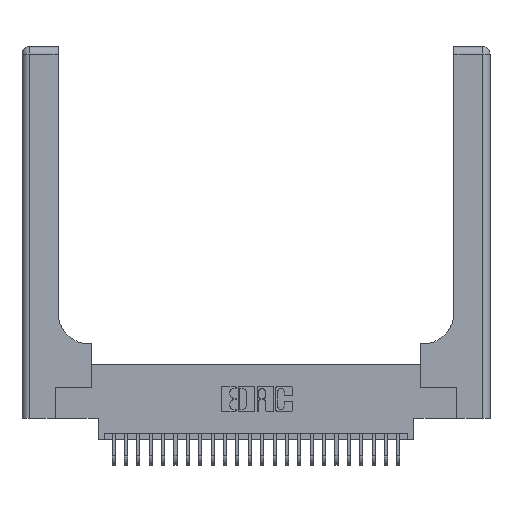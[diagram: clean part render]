
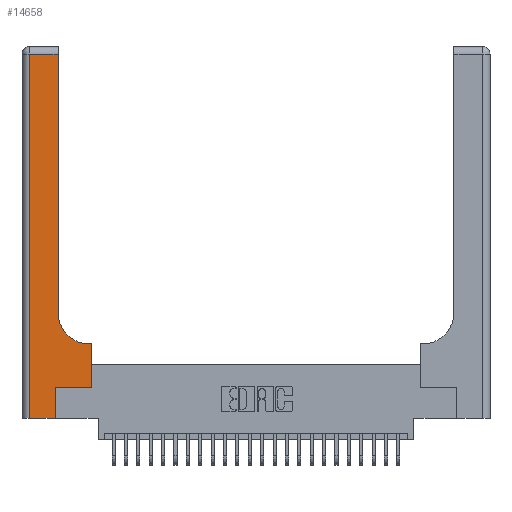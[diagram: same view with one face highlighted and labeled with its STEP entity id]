
A CAD part, top view. The second image highlights one B-rep face of the part: STEP entity #14658.
In plain terms, the highlighted planar face has unit normal (0, 0, 1).
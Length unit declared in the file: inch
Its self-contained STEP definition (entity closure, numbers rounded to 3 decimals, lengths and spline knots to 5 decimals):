
#450 = CARTESIAN_POINT ( 'NONE',  ( 0.06, 2.94, 0.37 ) ) ;
#3582 = LINE ( 'NONE', #26208, #14613 ) ;
#3914 = CARTESIAN_POINT ( 'NONE',  ( 0.2915, 2.94, 0.37 ) ) ;
#4185 = EDGE_CURVE ( 'NONE', #17432, #24767, #25683, .T. ) ;
#4216 = EDGE_CURVE ( 'NONE', #8321, #15777, #7664, .T. ) ;
#4225 = EDGE_CURVE ( 'NONE', #10453, #8321, #23656, .T. ) ;
#5013 = VERTEX_POINT ( 'NONE', #22377 ) ;
#6231 = ORIENTED_EDGE ( 'NONE', *, *, #25299, .T. ) ;
#6676 = DIRECTION ( 'NONE',  ( 0., 1., 0. ) ) ;
#6777 = CARTESIAN_POINT ( 'NONE',  ( 0.5415, 0.85, 0.37 ) ) ;
#6977 = VECTOR ( 'NONE', #6676, 39.37008 ) ;
#7330 = PLANE ( 'NONE',  #13040 ) ;
#7664 = LINE ( 'NONE', #8851, #6977 ) ;
#7935 = ORIENTED_EDGE ( 'NONE', *, *, #18161, .T. ) ;
#8321 = VERTEX_POINT ( 'NONE', #10564 ) ;
#8617 = VERTEX_POINT ( 'NONE', #15962 ) ;
#8851 = CARTESIAN_POINT ( 'NONE',  ( 0.2915, 3., 0.37 ) ) ;
#9047 = DIRECTION ( 'NONE',  ( 1., 0., 0. ) ) ;
#9924 = AXIS2_PLACEMENT_3D ( 'NONE', #6777, #22038, #9047 ) ;
#10279 = CARTESIAN_POINT ( 'NONE',  ( 0.5585, 0.6, 0.37 ) ) ;
#10350 = VECTOR ( 'NONE', #25368, 39.37008 ) ;
#10453 = VERTEX_POINT ( 'NONE', #26790 ) ;
#10564 = CARTESIAN_POINT ( 'NONE',  ( 0.2915, 0.85, 0.37 ) ) ;
#10685 = ORIENTED_EDGE ( 'NONE', *, *, #26089, .T. ) ;
#11084 = DIRECTION ( 'NONE',  ( 1., 0., 0. ) ) ;
#11159 = VERTEX_POINT ( 'NONE', #21205 ) ;
#11802 = DIRECTION ( 'NONE',  ( -1., 0., 0. ) ) ;
#12112 = VERTEX_POINT ( 'NONE', #450 ) ;
#12273 = DIRECTION ( 'NONE',  ( -1., 0., 0. ) ) ;
#12566 = LINE ( 'NONE', #24709, #23375 ) ;
#13028 = EDGE_CURVE ( 'NONE', #8617, #17432, #18296, .T. ) ;
#13040 = AXIS2_PLACEMENT_3D ( 'NONE', #22576, #24734, #11802 ) ;
#14613 = VECTOR ( 'NONE', #11084, 39.37008 ) ;
#14658 = ADVANCED_FACE ( 'NONE', ( #22779 ), #7330, .F. ) ;
#14773 = ORIENTED_EDGE ( 'NONE', *, *, #25739, .T. ) ;
#15777 = VERTEX_POINT ( 'NONE', #3914 ) ;
#15962 = CARTESIAN_POINT ( 'NONE',  ( 0.269, 0.25, 0.37 ) ) ;
#16182 = DIRECTION ( 'NONE',  ( 0., -1., 0. ) ) ;
#16433 = ORIENTED_EDGE ( 'NONE', *, *, #4216, .T. ) ;
#17313 = EDGE_LOOP ( 'NONE', ( #16433, #20477, #14773, #10685, #7935, #25943, #24284, #6231, #18461 ) ) ;
#17432 = VERTEX_POINT ( 'NONE', #21187 ) ;
#17570 = LINE ( 'NONE', #18905, #10350 ) ;
#18161 = EDGE_CURVE ( 'NONE', #5013, #8617, #18278, .T. ) ;
#18278 = LINE ( 'NONE', #19376, #19635 ) ;
#18296 = LINE ( 'NONE', #27711, #22649 ) ;
#18461 = ORIENTED_EDGE ( 'NONE', *, *, #4225, .T. ) ;
#18905 = CARTESIAN_POINT ( 'NONE',  ( 0., 2.94, 0.37 ) ) ;
#19311 = VECTOR ( 'NONE', #26077, 39.37008 ) ;
#19376 = CARTESIAN_POINT ( 'NONE',  ( 0.269, 0., 0.37 ) ) ;
#19635 = VECTOR ( 'NONE', #23678, 39.37008 ) ;
#20477 = ORIENTED_EDGE ( 'NONE', *, *, #21554, .T. ) ;
#20882 = CARTESIAN_POINT ( 'NONE',  ( 0.2915, 0.6, 0.37 ) ) ;
#21187 = CARTESIAN_POINT ( 'NONE',  ( 0.5585, 0.25, 0.37 ) ) ;
#21205 = CARTESIAN_POINT ( 'NONE',  ( 0.06, 0., 0.37 ) ) ;
#21554 = EDGE_CURVE ( 'NONE', #15777, #12112, #17570, .T. ) ;
#21758 = CARTESIAN_POINT ( 'NONE',  ( 0.5585, 0.25, 0.37 ) ) ;
#22038 = DIRECTION ( 'NONE',  ( 0., 0., -1. ) ) ;
#22377 = CARTESIAN_POINT ( 'NONE',  ( 0.269, 0., 0.37 ) ) ;
#22576 = CARTESIAN_POINT ( 'NONE',  ( 0., 3., 0.37 ) ) ;
#22649 = VECTOR ( 'NONE', #25664, 39.37008 ) ;
#22779 = FACE_OUTER_BOUND ( 'NONE', #17313, .T. ) ;
#23375 = VECTOR ( 'NONE', #16182, 39.37008 ) ;
#23656 = CIRCLE ( 'NONE', #9924, 0.25 ) ;
#23678 = DIRECTION ( 'NONE',  ( 0., 1., 0. ) ) ;
#24284 = ORIENTED_EDGE ( 'NONE', *, *, #4185, .T. ) ;
#24709 = CARTESIAN_POINT ( 'NONE',  ( 0.06, 3., 0.37 ) ) ;
#24734 = DIRECTION ( 'NONE',  ( 0., 0., -1. ) ) ;
#24767 = VERTEX_POINT ( 'NONE', #10279 ) ;
#25299 = EDGE_CURVE ( 'NONE', #24767, #10453, #28054, .T. ) ;
#25368 = DIRECTION ( 'NONE',  ( -1., 0., 0. ) ) ;
#25664 = DIRECTION ( 'NONE',  ( 1., 0., 0. ) ) ;
#25683 = LINE ( 'NONE', #21758, #19311 ) ;
#25739 = EDGE_CURVE ( 'NONE', #12112, #11159, #12566, .T. ) ;
#25943 = ORIENTED_EDGE ( 'NONE', *, *, #13028, .T. ) ;
#26077 = DIRECTION ( 'NONE',  ( 0., 1., 0. ) ) ;
#26089 = EDGE_CURVE ( 'NONE', #11159, #5013, #3582, .T. ) ;
#26208 = CARTESIAN_POINT ( 'NONE',  ( 0., 0., 0.37 ) ) ;
#26790 = CARTESIAN_POINT ( 'NONE',  ( 0.5415, 0.6, 0.37 ) ) ;
#27370 = VECTOR ( 'NONE', #12273, 39.37008 ) ;
#27711 = CARTESIAN_POINT ( 'NONE',  ( 0.269, 0.25, 0.37 ) ) ;
#28054 = LINE ( 'NONE', #20882, #27370 ) ;
